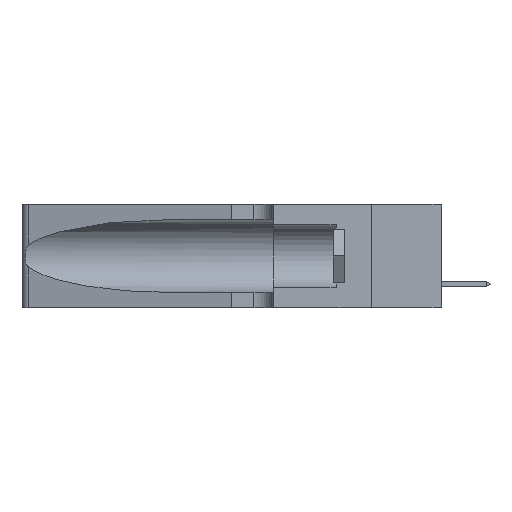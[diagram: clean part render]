
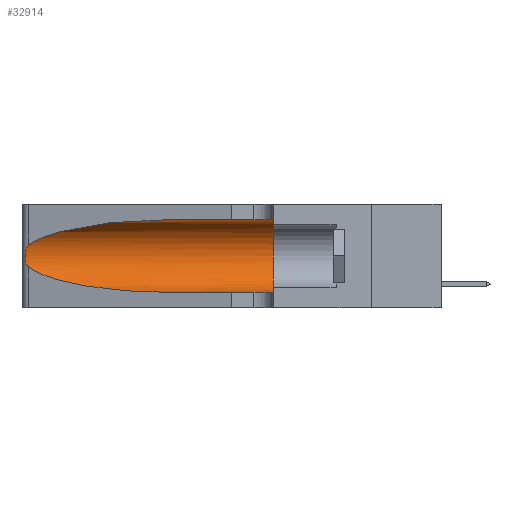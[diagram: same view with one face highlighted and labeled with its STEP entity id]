
A CAD part, left-side view. The second image highlights one B-rep face of the part: STEP entity #32914.
In plain terms, the highlighted cylindrical face has radius 3.308 mm (diameter 6.617 mm), a partial arc.
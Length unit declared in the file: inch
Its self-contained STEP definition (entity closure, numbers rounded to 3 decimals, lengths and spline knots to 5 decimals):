
#76 = CARTESIAN_POINT ( 'NONE',  ( 0.1305, 1.61858, 0.05475 ) ) ;
#605 = FACE_OUTER_BOUND ( 'NONE', #32572, .T. ) ;
#636 = CARTESIAN_POINT ( 'NONE',  ( 0.25789, 1.23486, 0.15765 ) ) ;
#836 = ORIENTED_EDGE ( 'NONE', *, *, #18255, .F. ) ;
#2510 = CARTESIAN_POINT ( 'NONE',  ( 0.1305, 0.35, 0.05475 ) ) ;
#3240 = VERTEX_POINT ( 'NONE', #13074 ) ;
#3481 = EDGE_CURVE ( 'NONE', #12556, #9857, #17051, .T. ) ;
#3804 = CARTESIAN_POINT ( 'NONE',  ( 0.26075, 1.23896, 0.178 ) ) ;
#4593 = DIRECTION ( 'NONE',  ( 0., 1., 0. ) ) ;
#5430 = CARTESIAN_POINT ( 'NONE',  ( 0.1305, 0.72297, 0.31525 ) ) ;
#6910 =( BOUNDED_CURVE ( )  B_SPLINE_CURVE ( 3, ( #25683, #22501, #13473, #37512 ),
 .UNSPECIFIED., .F., .T. ) 
 B_SPLINE_CURVE_WITH_KNOTS ( ( 4, 4 ),
 ( 1.5708, 2.84003 ),
 .UNSPECIFIED. ) 
 CURVE ( )  GEOMETRIC_REPRESENTATION_ITEM ( )  RATIONAL_B_SPLINE_CURVE ( ( 1., 0.87, 0.87, 1. ) ) 
 REPRESENTATION_ITEM ( '' )  );
#7288 = CIRCLE ( 'NONE', #18786, 0.13025 ) ;
#7555 = CARTESIAN_POINT ( 'NONE',  ( 0.1305, 0.35, 0.31525 ) ) ;
#7621 = AXIS2_PLACEMENT_3D ( 'NONE', #19072, #21945, #28046 ) ;
#9630 = ORIENTED_EDGE ( 'NONE', *, *, #38524, .T. ) ;
#9761 = B_SPLINE_CURVE_WITH_KNOTS ( 'NONE', 3,
 ( #35768, #35896, #21592, #37937, #20316, #36335, #12269, #3804, #24335, #18426, #636, #24575, #21425, #12666 ),
 .UNSPECIFIED., .F., .F.,
 ( 4, 2, 2, 2, 2, 2, 4 ),
 ( 0., 0.00027, 0.00053, 0.00107, 0.0016, 0.00187, 0.00214 ),
 .UNSPECIFIED. ) ;
#9857 = VERTEX_POINT ( 'NONE', #7555 ) ;
#11135 = EDGE_CURVE ( 'NONE', #13604, #11437, #38207, .T. ) ;
#11324 = ORIENTED_EDGE ( 'NONE', *, *, #3481, .F. ) ;
#11437 = VERTEX_POINT ( 'NONE', #23344 ) ;
#12269 = CARTESIAN_POINT ( 'NONE',  ( 0.26075, 1.23896, 0.19203 ) ) ;
#12556 = VERTEX_POINT ( 'NONE', #5430 ) ;
#12666 = CARTESIAN_POINT ( 'NONE',  ( 0.25487, 1.22718, 0.14631 ) ) ;
#12735 = DIRECTION ( 'NONE',  ( 0., -1., 0. ) ) ;
#13074 = CARTESIAN_POINT ( 'NONE',  ( 0.25487, 1.22718, 0.22369 ) ) ;
#13473 = CARTESIAN_POINT ( 'NONE',  ( 0.2373, 1.15595, 0.28018 ) ) ;
#13543 = CARTESIAN_POINT ( 'NONE',  ( 0.18966, 0.96281, 0.05475 ) ) ;
#13604 = VERTEX_POINT ( 'NONE', #25967 ) ;
#14679 = LINE ( 'NONE', #76, #16529 ) ;
#16529 = VECTOR ( 'NONE', #12735, 39.37008 ) ;
#16751 = CARTESIAN_POINT ( 'NONE',  ( 0.1305, 0.35, 0.185 ) ) ;
#17051 = LINE ( 'NONE', #23005, #18859 ) ;
#17104 = CARTESIAN_POINT ( 'NONE',  ( 0.2373, 1.15595, 0.08982 ) ) ;
#18255 = EDGE_CURVE ( 'NONE', #9857, #23354, #7288, .T. ) ;
#18367 = ORIENTED_EDGE ( 'NONE', *, *, #28961, .T. ) ;
#18400 = CYLINDRICAL_SURFACE ( 'NONE', #7621, 0.13025 ) ;
#18426 = CARTESIAN_POINT ( 'NONE',  ( 0.25856, 1.23593, 0.16098 ) ) ;
#18786 = AXIS2_PLACEMENT_3D ( 'NONE', #16751, #4593, #19490 ) ;
#18859 = VECTOR ( 'NONE', #32338, 39.37008 ) ;
#19072 = CARTESIAN_POINT ( 'NONE',  ( 0.1305, 1.61858, 0.185 ) ) ;
#19490 = DIRECTION ( 'NONE',  ( 0., 0., 1. ) ) ;
#20316 = CARTESIAN_POINT ( 'NONE',  ( 0.25854, 1.2359, 0.20912 ) ) ;
#21425 = CARTESIAN_POINT ( 'NONE',  ( 0.25555, 1.22993, 0.14849 ) ) ;
#21592 = CARTESIAN_POINT ( 'NONE',  ( 0.25639, 1.23184, 0.21858 ) ) ;
#21887 = CARTESIAN_POINT ( 'NONE',  ( 0.25487, 1.22718, 0.14631 ) ) ;
#21945 = DIRECTION ( 'NONE',  ( 0., -1., 0. ) ) ;
#22501 = CARTESIAN_POINT ( 'NONE',  ( 0.18966, 0.96281, 0.31525 ) ) ;
#23005 = CARTESIAN_POINT ( 'NONE',  ( 0.1305, 1.61858, 0.31525 ) ) ;
#23344 = CARTESIAN_POINT ( 'NONE',  ( 0.1305, 0.72297, 0.05475 ) ) ;
#23354 = VERTEX_POINT ( 'NONE', #2510 ) ;
#24335 = CARTESIAN_POINT ( 'NONE',  ( 0.26017, 1.23833, 0.17102 ) ) ;
#24575 = CARTESIAN_POINT ( 'NONE',  ( 0.25639, 1.23186, 0.15144 ) ) ;
#25178 = CARTESIAN_POINT ( 'NONE',  ( 0.1305, 0.72297, 0.05475 ) ) ;
#25683 = CARTESIAN_POINT ( 'NONE',  ( 0.1305, 0.72297, 0.31525 ) ) ;
#25967 = CARTESIAN_POINT ( 'NONE',  ( 0.25487, 1.22718, 0.14631 ) ) ;
#28046 = DIRECTION ( 'NONE',  ( 0., 0., -1. ) ) ;
#28961 = EDGE_CURVE ( 'NONE', #3240, #13604, #9761, .T. ) ;
#29357 = ORIENTED_EDGE ( 'NONE', *, *, #37525, .T. ) ;
#32338 = DIRECTION ( 'NONE',  ( 0., -1., 0. ) ) ;
#32572 = EDGE_LOOP ( 'NONE', ( #29357, #18367, #35805, #9630, #836, #11324 ) ) ;
#32914 = ADVANCED_FACE ( 'NONE', ( #605 ), #18400, .F. ) ;
#35768 = CARTESIAN_POINT ( 'NONE',  ( 0.25487, 1.22718, 0.22369 ) ) ;
#35805 = ORIENTED_EDGE ( 'NONE', *, *, #11135, .T. ) ;
#35896 = CARTESIAN_POINT ( 'NONE',  ( 0.25555, 1.22994, 0.2215 ) ) ;
#36335 = CARTESIAN_POINT ( 'NONE',  ( 0.26018, 1.23835, 0.19895 ) ) ;
#37512 = CARTESIAN_POINT ( 'NONE',  ( 0.25487, 1.22718, 0.22369 ) ) ;
#37525 = EDGE_CURVE ( 'NONE', #12556, #3240, #6910, .T. ) ;
#37937 = CARTESIAN_POINT ( 'NONE',  ( 0.25787, 1.23484, 0.2124 ) ) ;
#38207 =( BOUNDED_CURVE ( )  B_SPLINE_CURVE ( 3, ( #21887, #17104, #13543, #25178 ),
 .UNSPECIFIED., .F., .T. ) 
 B_SPLINE_CURVE_WITH_KNOTS ( ( 4, 4 ),
 ( 3.44316, 4.71239 ),
 .UNSPECIFIED. ) 
 CURVE ( )  GEOMETRIC_REPRESENTATION_ITEM ( )  RATIONAL_B_SPLINE_CURVE ( ( 1., 0.87, 0.87, 1. ) ) 
 REPRESENTATION_ITEM ( '' )  );
#38524 = EDGE_CURVE ( 'NONE', #11437, #23354, #14679, .T. ) ;
